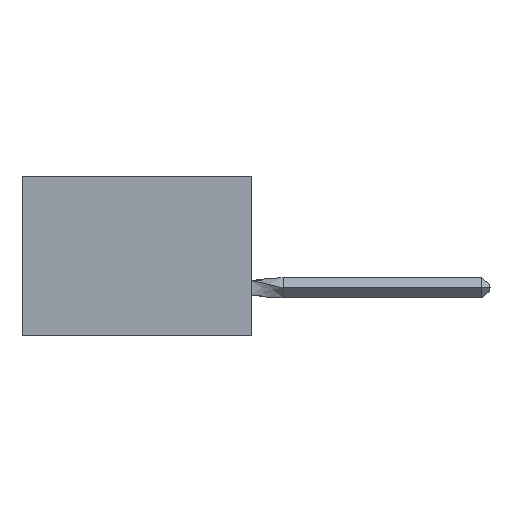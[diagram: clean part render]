
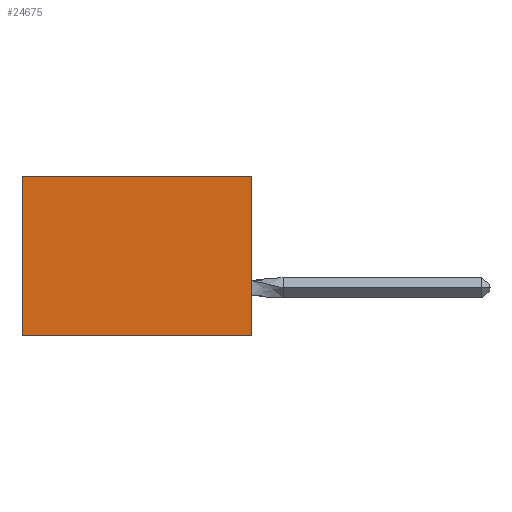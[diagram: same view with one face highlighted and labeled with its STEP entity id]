
A CAD part, left-side view. The second image highlights one B-rep face of the part: STEP entity #24675.
In plain terms, the highlighted planar face has unit normal (-1, 0, 0).
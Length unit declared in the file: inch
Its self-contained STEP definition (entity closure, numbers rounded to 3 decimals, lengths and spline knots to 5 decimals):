
#1256 = VECTOR ( 'NONE', #40616, 39.37008 ) ;
#3443 = VERTEX_POINT ( 'NONE', #44490 ) ;
#3998 = ORIENTED_EDGE ( 'NONE', *, *, #15123, .F. ) ;
#5702 = DIRECTION ( 'NONE',  ( 1., 0., 0. ) ) ;
#5846 = CARTESIAN_POINT ( 'NONE',  ( 0.305, 0., -0.5 ) ) ;
#6041 = CARTESIAN_POINT ( 'NONE',  ( 0.305, 0.72, -0.5 ) ) ;
#6615 = LINE ( 'NONE', #34685, #33989 ) ;
#6687 = DIRECTION ( 'NONE',  ( 0., 0., -1. ) ) ;
#7220 = CARTESIAN_POINT ( 'NONE',  ( 0.305, 0., -0.5 ) ) ;
#13250 = FACE_OUTER_BOUND ( 'NONE', #17136, .T. ) ;
#13497 = VERTEX_POINT ( 'NONE', #28458 ) ;
#14368 = EDGE_CURVE ( 'NONE', #3443, #35443, #26393, .T. ) ;
#15123 = EDGE_CURVE ( 'NONE', #13497, #3443, #38068, .T. ) ;
#16476 = DIRECTION ( 'NONE',  ( 0., 0., -1. ) ) ;
#17136 = EDGE_LOOP ( 'NONE', ( #37099, #19052, #3998, #25693 ) ) ;
#17509 = VECTOR ( 'NONE', #32098, 39.37008 ) ;
#19052 = ORIENTED_EDGE ( 'NONE', *, *, #14368, .F. ) ;
#22541 = LINE ( 'NONE', #39027, #17509 ) ;
#22747 = CARTESIAN_POINT ( 'NONE',  ( 0.305, 0., -0.5 ) ) ;
#23384 = AXIS2_PLACEMENT_3D ( 'NONE', #5846, #5702, #16476 ) ;
#23976 = PLANE ( 'NONE',  #23384 ) ;
#24675 = ADVANCED_FACE ( 'NONE', ( #13250 ), #23976, .F. ) ;
#25233 = CARTESIAN_POINT ( 'NONE',  ( 0.305, 0.72, 0. ) ) ;
#25693 = ORIENTED_EDGE ( 'NONE', *, *, #34181, .T. ) ;
#25721 = VERTEX_POINT ( 'NONE', #25233 ) ;
#26393 = LINE ( 'NONE', #22747, #1256 ) ;
#27712 = EDGE_CURVE ( 'NONE', #25721, #35443, #6615, .T. ) ;
#28420 = DIRECTION ( 'NONE',  ( 0., 0., -1. ) ) ;
#28458 = CARTESIAN_POINT ( 'NONE',  ( 0.305, 0., 0. ) ) ;
#32098 = DIRECTION ( 'NONE',  ( 0., 1., 0. ) ) ;
#33989 = VECTOR ( 'NONE', #6687, 39.37008 ) ;
#34181 = EDGE_CURVE ( 'NONE', #13497, #25721, #22541, .T. ) ;
#34685 = CARTESIAN_POINT ( 'NONE',  ( 0.305, 0.72, -0.5 ) ) ;
#35443 = VERTEX_POINT ( 'NONE', #6041 ) ;
#37099 = ORIENTED_EDGE ( 'NONE', *, *, #27712, .T. ) ;
#38068 = LINE ( 'NONE', #7220, #40948 ) ;
#39027 = CARTESIAN_POINT ( 'NONE',  ( 0.305, 0., 0. ) ) ;
#40616 = DIRECTION ( 'NONE',  ( 0., 1., 0. ) ) ;
#40948 = VECTOR ( 'NONE', #28420, 39.37008 ) ;
#44490 = CARTESIAN_POINT ( 'NONE',  ( 0.305, 0., -0.5 ) ) ;
